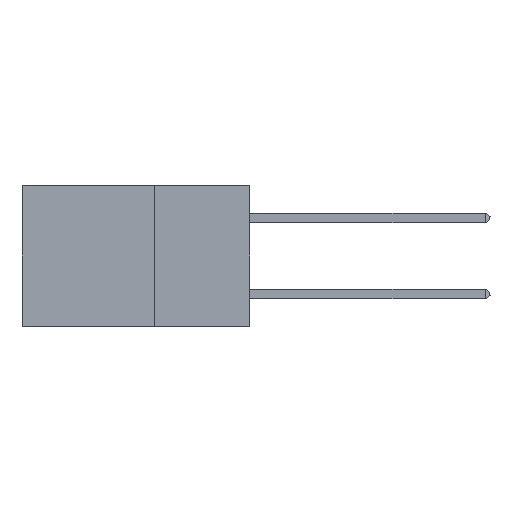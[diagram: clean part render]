
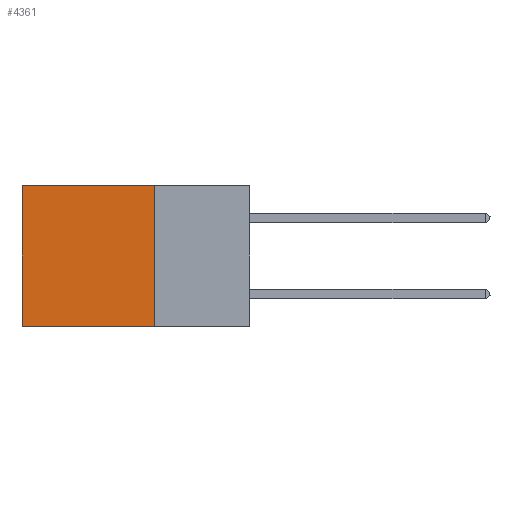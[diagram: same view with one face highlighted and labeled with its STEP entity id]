
A CAD part, left-side view. The second image highlights one B-rep face of the part: STEP entity #4361.
In plain terms, the highlighted planar face has unit normal (-1, 0, 0).
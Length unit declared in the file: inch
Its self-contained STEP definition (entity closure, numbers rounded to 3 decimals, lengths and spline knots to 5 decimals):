
#8 = DIRECTION ( 'NONE',  ( 0., 0., -1. ) ) ;
#1788 = CARTESIAN_POINT ( 'NONE',  ( 0.2875, 0.25, 0. ) ) ;
#1801 = CARTESIAN_POINT ( 'NONE',  ( 0.2875, 0.6, -0.37 ) ) ;
#1980 = CARTESIAN_POINT ( 'NONE',  ( 0.2875, 0.6, 0. ) ) ;
#2465 = CARTESIAN_POINT ( 'NONE',  ( 0.2875, 0.25, 0. ) ) ;
#2873 = VECTOR ( 'NONE', #21253, 39.37008 ) ;
#3138 = EDGE_LOOP ( 'NONE', ( #5313, #17388, #9886, #3596 ) ) ;
#3215 = CARTESIAN_POINT ( 'NONE',  ( 0.2875, 0.25, 0. ) ) ;
#3559 = VECTOR ( 'NONE', #10623, 39.37008 ) ;
#3596 = ORIENTED_EDGE ( 'NONE', *, *, #10602, .T. ) ;
#3781 = DIRECTION ( 'NONE',  ( 0., 0., -1. ) ) ;
#4312 = DIRECTION ( 'NONE',  ( 1., 0., 0. ) ) ;
#4361 = ADVANCED_FACE ( 'NONE', ( #14825 ), #11874, .F. ) ;
#5313 = ORIENTED_EDGE ( 'NONE', *, *, #9782, .T. ) ;
#6276 = LINE ( 'NONE', #1980, #11283 ) ;
#8455 = VERTEX_POINT ( 'NONE', #17828 ) ;
#8523 = EDGE_CURVE ( 'NONE', #8455, #17289, #18631, .T. ) ;
#8636 = CARTESIAN_POINT ( 'NONE',  ( 0.2875, 0.6, 0. ) ) ;
#9782 = EDGE_CURVE ( 'NONE', #19403, #17289, #6276, .T. ) ;
#9886 = ORIENTED_EDGE ( 'NONE', *, *, #13108, .F. ) ;
#10602 = EDGE_CURVE ( 'NONE', #12319, #19403, #22270, .T. ) ;
#10623 = DIRECTION ( 'NONE',  ( 0., 1., 0. ) ) ;
#11227 = LINE ( 'NONE', #1788, #21112 ) ;
#11283 = VECTOR ( 'NONE', #8, 39.37008 ) ;
#11874 = PLANE ( 'NONE',  #16643 ) ;
#12319 = VERTEX_POINT ( 'NONE', #3215 ) ;
#13108 = EDGE_CURVE ( 'NONE', #12319, #8455, #11227, .T. ) ;
#14825 = FACE_OUTER_BOUND ( 'NONE', #3138, .T. ) ;
#15644 = CARTESIAN_POINT ( 'NONE',  ( 0.2875, 0.25, 0. ) ) ;
#16643 = AXIS2_PLACEMENT_3D ( 'NONE', #15644, #4312, #17518 ) ;
#17289 = VERTEX_POINT ( 'NONE', #1801 ) ;
#17388 = ORIENTED_EDGE ( 'NONE', *, *, #8523, .F. ) ;
#17518 = DIRECTION ( 'NONE',  ( 0., 0., -1. ) ) ;
#17828 = CARTESIAN_POINT ( 'NONE',  ( 0.2875, 0.25, -0.37 ) ) ;
#18631 = LINE ( 'NONE', #19923, #3559 ) ;
#19403 = VERTEX_POINT ( 'NONE', #8636 ) ;
#19923 = CARTESIAN_POINT ( 'NONE',  ( 0.2875, 0.25, -0.37 ) ) ;
#21112 = VECTOR ( 'NONE', #3781, 39.37008 ) ;
#21253 = DIRECTION ( 'NONE',  ( 0., 1., 0. ) ) ;
#22270 = LINE ( 'NONE', #2465, #2873 ) ;
